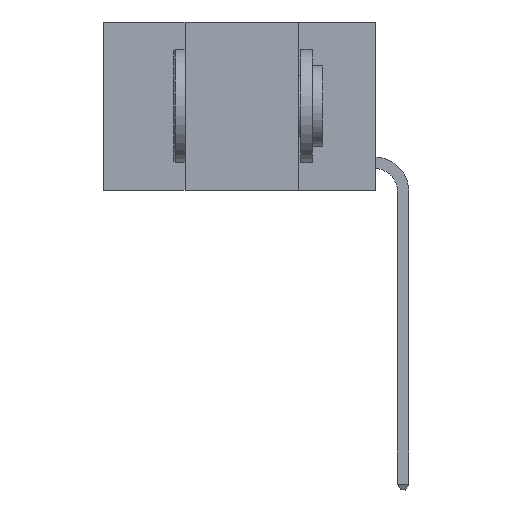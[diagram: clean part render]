
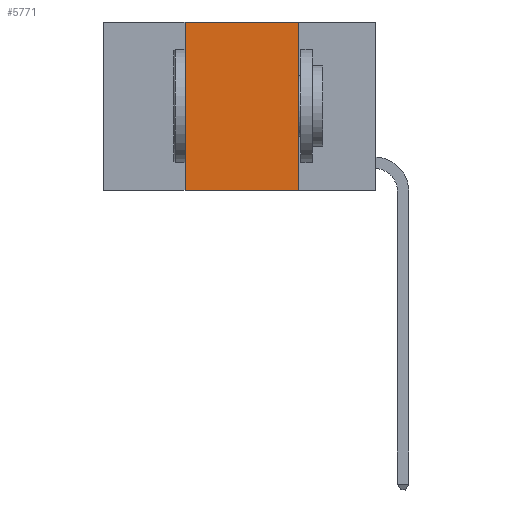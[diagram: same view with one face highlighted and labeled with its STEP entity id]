
A CAD part, left-side view. The second image highlights one B-rep face of the part: STEP entity #5771.
In plain terms, the highlighted planar face has unit normal (-1, 0, 0).
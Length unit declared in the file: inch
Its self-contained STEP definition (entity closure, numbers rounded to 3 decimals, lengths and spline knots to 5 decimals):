
#174 = DIRECTION ( 'NONE',  ( 0., -1., 0. ) ) ;
#304 = ORIENTED_EDGE ( 'NONE', *, *, #18493, .F. ) ;
#307 = VECTOR ( 'NONE', #174, 39.37008 ) ;
#2623 = ORIENTED_EDGE ( 'NONE', *, *, #17859, .T. ) ;
#2740 = CARTESIAN_POINT ( 'NONE',  ( 0., 0.17, -0.37 ) ) ;
#2839 = PLANE ( 'NONE',  #3164 ) ;
#3036 = LINE ( 'NONE', #9046, #10206 ) ;
#3164 = AXIS2_PLACEMENT_3D ( 'NONE', #12911, #5778, #15818 ) ;
#3768 = LINE ( 'NONE', #7561, #7582 ) ;
#3947 = CARTESIAN_POINT ( 'NONE',  ( 0., 0.42, -0.37 ) ) ;
#4262 = ORIENTED_EDGE ( 'NONE', *, *, #16937, .F. ) ;
#5615 = EDGE_LOOP ( 'NONE', ( #304, #6431, #4262, #2623 ) ) ;
#5771 = ADVANCED_FACE ( 'NONE', ( #8014 ), #2839, .F. ) ;
#5778 = DIRECTION ( 'NONE',  ( 1., 0., 0. ) ) ;
#6431 = ORIENTED_EDGE ( 'NONE', *, *, #16252, .F. ) ;
#6635 = VECTOR ( 'NONE', #9071, 39.37008 ) ;
#7561 = CARTESIAN_POINT ( 'NONE',  ( 0., 0.42, 0. ) ) ;
#7582 = VECTOR ( 'NONE', #17617, 39.37008 ) ;
#8014 = FACE_OUTER_BOUND ( 'NONE', #5615, .T. ) ;
#8030 = LINE ( 'NONE', #13132, #307 ) ;
#9046 = CARTESIAN_POINT ( 'NONE',  ( 0., 0.17, 0. ) ) ;
#9071 = DIRECTION ( 'NONE',  ( 0., -1., 0. ) ) ;
#10206 = VECTOR ( 'NONE', #10485, 39.37008 ) ;
#10485 = DIRECTION ( 'NONE',  ( 0., 0., -1. ) ) ;
#10591 = VERTEX_POINT ( 'NONE', #2740 ) ;
#11456 = VERTEX_POINT ( 'NONE', #12138 ) ;
#12138 = CARTESIAN_POINT ( 'NONE',  ( 0., 0.42, 0. ) ) ;
#12672 = VERTEX_POINT ( 'NONE', #16793 ) ;
#12911 = CARTESIAN_POINT ( 'NONE',  ( 0., 0.6, 0. ) ) ;
#13132 = CARTESIAN_POINT ( 'NONE',  ( 0., 0.6, 0. ) ) ;
#13829 = VERTEX_POINT ( 'NONE', #3947 ) ;
#14312 = LINE ( 'NONE', #17687, #6635 ) ;
#15818 = DIRECTION ( 'NONE',  ( 0., 0., -1. ) ) ;
#16252 = EDGE_CURVE ( 'NONE', #11456, #12672, #8030, .T. ) ;
#16793 = CARTESIAN_POINT ( 'NONE',  ( 0., 0.17, 0. ) ) ;
#16937 = EDGE_CURVE ( 'NONE', #13829, #11456, #3768, .T. ) ;
#17617 = DIRECTION ( 'NONE',  ( 0., 0., 1. ) ) ;
#17687 = CARTESIAN_POINT ( 'NONE',  ( 0., 0.6, -0.37 ) ) ;
#17859 = EDGE_CURVE ( 'NONE', #13829, #10591, #14312, .T. ) ;
#18493 = EDGE_CURVE ( 'NONE', #12672, #10591, #3036, .T. ) ;
